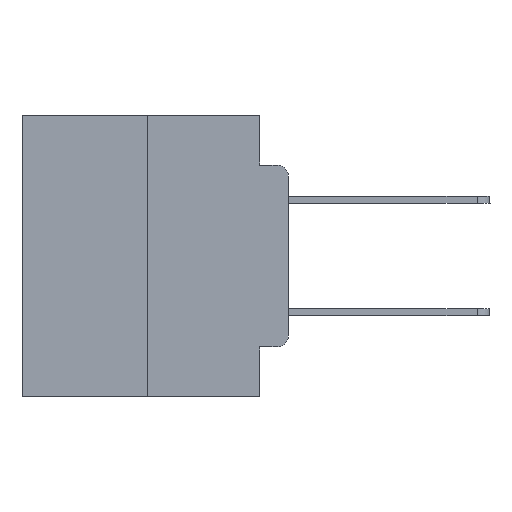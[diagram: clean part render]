
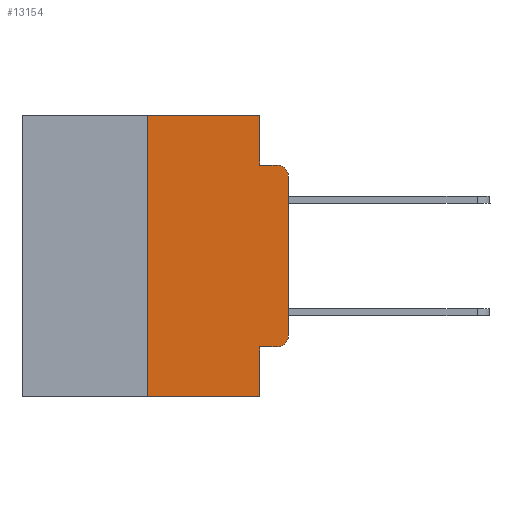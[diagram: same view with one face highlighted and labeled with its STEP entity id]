
A CAD part, left-side view. The second image highlights one B-rep face of the part: STEP entity #13154.
In plain terms, the highlighted planar face has unit normal (-1, 0, 0).
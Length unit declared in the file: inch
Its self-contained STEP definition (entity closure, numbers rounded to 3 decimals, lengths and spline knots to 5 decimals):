
#534 = VECTOR ( 'NONE', #9115, 39.37008 ) ;
#1282 = EDGE_CURVE ( 'NONE', #26062, #18391, #8282, .T. ) ;
#1462 = LINE ( 'NONE', #17091, #15882 ) ;
#1538 = VERTEX_POINT ( 'NONE', #4183 ) ;
#1864 = CARTESIAN_POINT ( 'NONE',  ( 0., 0.25, -0.5 ) ) ;
#2551 = CARTESIAN_POINT ( 'NONE',  ( 0., 0.051, -0.4115 ) ) ;
#2827 = CARTESIAN_POINT ( 'NONE',  ( 0., 0.051, 0. ) ) ;
#2956 = CARTESIAN_POINT ( 'NONE',  ( 0., 0., -0.3915 ) ) ;
#3008 = VECTOR ( 'NONE', #27388, 39.37008 ) ;
#4183 = CARTESIAN_POINT ( 'NONE',  ( 0., 0.051, -0.5 ) ) ;
#4441 = EDGE_CURVE ( 'NONE', #23427, #26139, #28371, .T. ) ;
#4637 = ORIENTED_EDGE ( 'NONE', *, *, #13675, .F. ) ;
#4918 = ORIENTED_EDGE ( 'NONE', *, *, #1282, .T. ) ;
#5739 = DIRECTION ( 'NONE',  ( 0., 0., -1. ) ) ;
#6044 = CARTESIAN_POINT ( 'NONE',  ( 0., 0.02, -0.4115 ) ) ;
#6358 = VECTOR ( 'NONE', #12904, 39.37008 ) ;
#6380 = CARTESIAN_POINT ( 'NONE',  ( 0., 0.25, 0. ) ) ;
#6401 = DIRECTION ( 'NONE',  ( 0., -1., 0. ) ) ;
#6656 = CARTESIAN_POINT ( 'NONE',  ( 0., 0.051, -0.0885 ) ) ;
#6757 = CIRCLE ( 'NONE', #12298, 0.02 ) ;
#7336 = DIRECTION ( 'NONE',  ( 0., 0., -1. ) ) ;
#7544 = DIRECTION ( 'NONE',  ( -1., 0., 0. ) ) ;
#8074 = CIRCLE ( 'NONE', #16800, 0.02 ) ;
#8282 = LINE ( 'NONE', #10305, #20110 ) ;
#9115 = DIRECTION ( 'NONE',  ( 0., -1., 0. ) ) ;
#9324 = EDGE_CURVE ( 'NONE', #11034, #13119, #13175, .T. ) ;
#9650 = VECTOR ( 'NONE', #5739, 39.37008 ) ;
#9757 = LINE ( 'NONE', #20593, #3008 ) ;
#10237 = CARTESIAN_POINT ( 'NONE',  ( 0., 0.051, -0.0885 ) ) ;
#10305 = CARTESIAN_POINT ( 'NONE',  ( 0., 0.051, -0.4115 ) ) ;
#10462 = DIRECTION ( 'NONE',  ( -1., 0., 0. ) ) ;
#10737 = LINE ( 'NONE', #19550, #23382 ) ;
#11017 = ORIENTED_EDGE ( 'NONE', *, *, #25258, .T. ) ;
#11034 = VERTEX_POINT ( 'NONE', #10237 ) ;
#12155 = LINE ( 'NONE', #18521, #28322 ) ;
#12169 = CARTESIAN_POINT ( 'NONE',  ( 0., 0.02, -0.3915 ) ) ;
#12298 = AXIS2_PLACEMENT_3D ( 'NONE', #12169, #7544, #23436 ) ;
#12570 = ORIENTED_EDGE ( 'NONE', *, *, #18960, .F. ) ;
#12904 = DIRECTION ( 'NONE',  ( 0., 0., 1. ) ) ;
#13119 = VERTEX_POINT ( 'NONE', #22505 ) ;
#13154 = ADVANCED_FACE ( 'NONE', ( #24976 ), #18752, .F. ) ;
#13175 = LINE ( 'NONE', #6656, #534 ) ;
#13294 = EDGE_CURVE ( 'NONE', #19567, #13119, #8074, .T. ) ;
#13675 = EDGE_CURVE ( 'NONE', #26139, #23991, #1462, .T. ) ;
#14937 = DIRECTION ( 'NONE',  ( 0., -1., 0. ) ) ;
#14944 = EDGE_CURVE ( 'NONE', #26062, #1538, #9757, .T. ) ;
#15678 = ORIENTED_EDGE ( 'NONE', *, *, #22003, .T. ) ;
#15882 = VECTOR ( 'NONE', #19395, 39.37008 ) ;
#16017 = CARTESIAN_POINT ( 'NONE',  ( 0., 0.473, 0. ) ) ;
#16411 = EDGE_CURVE ( 'NONE', #23427, #1538, #10737, .T. ) ;
#16429 = CARTESIAN_POINT ( 'NONE',  ( 0., 0.051, 0. ) ) ;
#16590 = DIRECTION ( 'NONE',  ( 0., 0., -1. ) ) ;
#16800 = AXIS2_PLACEMENT_3D ( 'NONE', #24047, #10462, #16590 ) ;
#17091 = CARTESIAN_POINT ( 'NONE',  ( 0., 0.473, 0. ) ) ;
#18391 = VERTEX_POINT ( 'NONE', #6044 ) ;
#18521 = CARTESIAN_POINT ( 'NONE',  ( 0., 0., 0. ) ) ;
#18752 = PLANE ( 'NONE',  #25103 ) ;
#18960 = EDGE_CURVE ( 'NONE', #23991, #11034, #19161, .T. ) ;
#19161 = LINE ( 'NONE', #16429, #9650 ) ;
#19395 = DIRECTION ( 'NONE',  ( 0., -1., 0. ) ) ;
#19550 = CARTESIAN_POINT ( 'NONE',  ( 0., 0.473, -0.5 ) ) ;
#19567 = VERTEX_POINT ( 'NONE', #26749 ) ;
#20110 = VECTOR ( 'NONE', #14937, 39.37008 ) ;
#20389 = DIRECTION ( 'NONE',  ( 0., 0., 1. ) ) ;
#20593 = CARTESIAN_POINT ( 'NONE',  ( 0., 0.051, 0. ) ) ;
#21127 = VERTEX_POINT ( 'NONE', #2956 ) ;
#21328 = ORIENTED_EDGE ( 'NONE', *, *, #13294, .T. ) ;
#21356 = ORIENTED_EDGE ( 'NONE', *, *, #16411, .T. ) ;
#22003 = EDGE_CURVE ( 'NONE', #21127, #19567, #12155, .T. ) ;
#22505 = CARTESIAN_POINT ( 'NONE',  ( 0., 0.02, -0.0885 ) ) ;
#22907 = ORIENTED_EDGE ( 'NONE', *, *, #4441, .F. ) ;
#23382 = VECTOR ( 'NONE', #6401, 39.37008 ) ;
#23427 = VERTEX_POINT ( 'NONE', #1864 ) ;
#23436 = DIRECTION ( 'NONE',  ( 0., 0., -1. ) ) ;
#23991 = VERTEX_POINT ( 'NONE', #2827 ) ;
#24047 = CARTESIAN_POINT ( 'NONE',  ( 0., 0.02, -0.1085 ) ) ;
#24349 = EDGE_LOOP ( 'NONE', ( #15678, #21328, #26405, #12570, #4637, #22907, #21356, #28091, #4918, #11017 ) ) ;
#24976 = FACE_OUTER_BOUND ( 'NONE', #24349, .T. ) ;
#25103 = AXIS2_PLACEMENT_3D ( 'NONE', #16017, #27570, #7336 ) ;
#25256 = CARTESIAN_POINT ( 'NONE',  ( 0., 0.25, 0. ) ) ;
#25258 = EDGE_CURVE ( 'NONE', #18391, #21127, #6757, .T. ) ;
#26062 = VERTEX_POINT ( 'NONE', #2551 ) ;
#26139 = VERTEX_POINT ( 'NONE', #25256 ) ;
#26405 = ORIENTED_EDGE ( 'NONE', *, *, #9324, .F. ) ;
#26749 = CARTESIAN_POINT ( 'NONE',  ( 0., 0., -0.1085 ) ) ;
#27388 = DIRECTION ( 'NONE',  ( 0., 0., -1. ) ) ;
#27570 = DIRECTION ( 'NONE',  ( 1., 0., 0. ) ) ;
#28091 = ORIENTED_EDGE ( 'NONE', *, *, #14944, .F. ) ;
#28322 = VECTOR ( 'NONE', #20389, 39.37008 ) ;
#28371 = LINE ( 'NONE', #6380, #6358 ) ;
